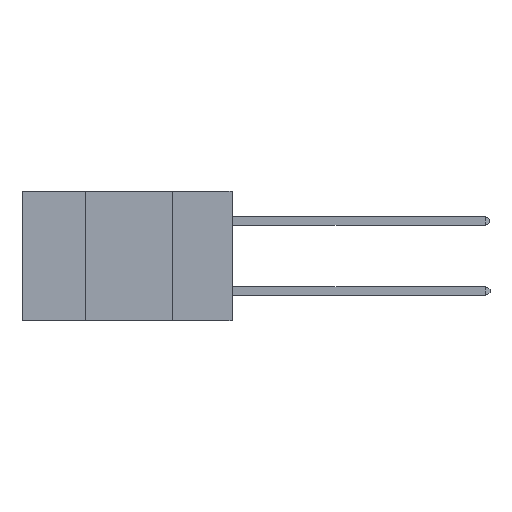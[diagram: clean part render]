
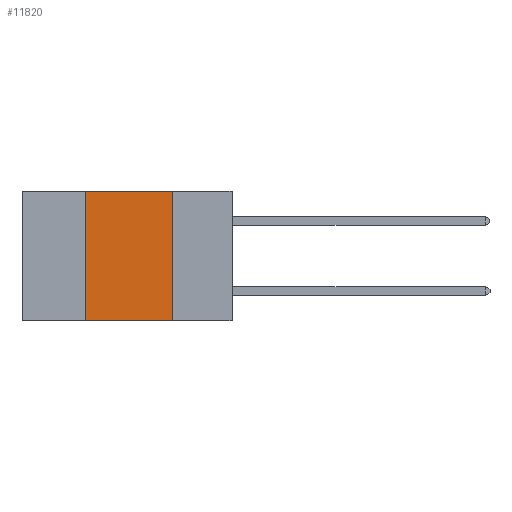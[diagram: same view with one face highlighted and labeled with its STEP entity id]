
A CAD part, left-side view. The second image highlights one B-rep face of the part: STEP entity #11820.
In plain terms, the highlighted planar face has unit normal (-1, 0, 0).
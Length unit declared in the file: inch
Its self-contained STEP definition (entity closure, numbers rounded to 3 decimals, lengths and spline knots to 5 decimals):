
#754 = LINE ( 'NONE', #2437, #10613 ) ;
#2350 = CARTESIAN_POINT ( 'NONE',  ( 0., 0.17, 0. ) ) ;
#2437 = CARTESIAN_POINT ( 'NONE',  ( 0., 0.6, 0. ) ) ;
#3886 = VECTOR ( 'NONE', #15499, 39.37008 ) ;
#4356 = DIRECTION ( 'NONE',  ( 0., 0., 1. ) ) ;
#4538 = VERTEX_POINT ( 'NONE', #9562 ) ;
#4907 = VERTEX_POINT ( 'NONE', #14312 ) ;
#5766 = EDGE_LOOP ( 'NONE', ( #22952, #10340, #20429, #6708 ) ) ;
#5913 = FACE_OUTER_BOUND ( 'NONE', #5766, .T. ) ;
#5994 = EDGE_CURVE ( 'NONE', #4538, #4907, #9870, .T. ) ;
#6028 = VECTOR ( 'NONE', #4356, 39.37008 ) ;
#6362 = DIRECTION ( 'NONE',  ( 0., -1., 0. ) ) ;
#6708 = ORIENTED_EDGE ( 'NONE', *, *, #5994, .T. ) ;
#8091 = PLANE ( 'NONE',  #16454 ) ;
#9562 = CARTESIAN_POINT ( 'NONE',  ( 0., 0.42, -0.37 ) ) ;
#9870 = LINE ( 'NONE', #17137, #15262 ) ;
#9916 = DIRECTION ( 'NONE',  ( 1., 0., 0. ) ) ;
#9921 = DIRECTION ( 'NONE',  ( 0., -1., 0. ) ) ;
#10340 = ORIENTED_EDGE ( 'NONE', *, *, #14292, .F. ) ;
#10497 = EDGE_CURVE ( 'NONE', #4538, #19419, #19230, .T. ) ;
#10613 = VECTOR ( 'NONE', #9921, 39.37008 ) ;
#11257 = EDGE_CURVE ( 'NONE', #16033, #4907, #18314, .T. ) ;
#11820 = ADVANCED_FACE ( 'NONE', ( #5913 ), #8091, .F. ) ;
#13675 = CARTESIAN_POINT ( 'NONE',  ( 0., 0.17, 0. ) ) ;
#14292 = EDGE_CURVE ( 'NONE', #19419, #16033, #754, .T. ) ;
#14312 = CARTESIAN_POINT ( 'NONE',  ( 0., 0.17, -0.37 ) ) ;
#15262 = VECTOR ( 'NONE', #6362, 39.37008 ) ;
#15286 = CARTESIAN_POINT ( 'NONE',  ( 0., 0.42, 0. ) ) ;
#15499 = DIRECTION ( 'NONE',  ( 0., 0., -1. ) ) ;
#16033 = VERTEX_POINT ( 'NONE', #2350 ) ;
#16454 = AXIS2_PLACEMENT_3D ( 'NONE', #20654, #9916, #22442 ) ;
#17137 = CARTESIAN_POINT ( 'NONE',  ( 0., 0.6, -0.37 ) ) ;
#17222 = CARTESIAN_POINT ( 'NONE',  ( 0., 0.42, 0. ) ) ;
#18314 = LINE ( 'NONE', #13675, #3886 ) ;
#19230 = LINE ( 'NONE', #15286, #6028 ) ;
#19419 = VERTEX_POINT ( 'NONE', #17222 ) ;
#20429 = ORIENTED_EDGE ( 'NONE', *, *, #10497, .F. ) ;
#20654 = CARTESIAN_POINT ( 'NONE',  ( 0., 0.6, 0. ) ) ;
#22442 = DIRECTION ( 'NONE',  ( 0., 0., -1. ) ) ;
#22952 = ORIENTED_EDGE ( 'NONE', *, *, #11257, .F. ) ;
